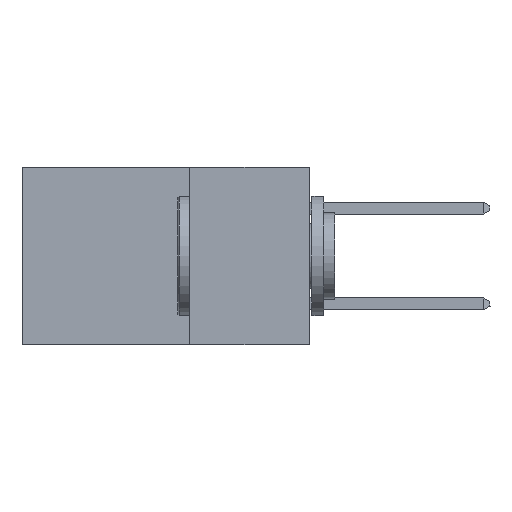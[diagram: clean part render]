
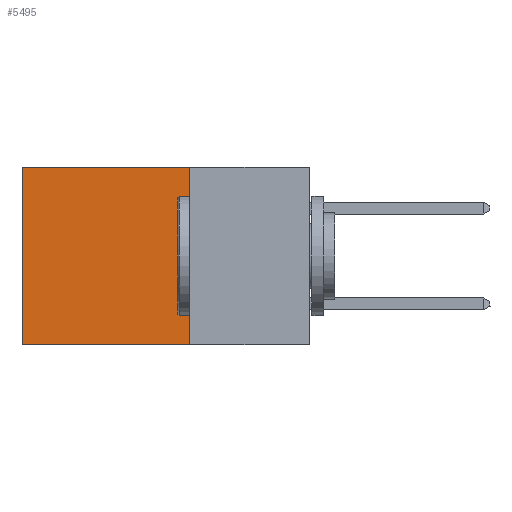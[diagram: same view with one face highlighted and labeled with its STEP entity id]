
A CAD part, left-side view. The second image highlights one B-rep face of the part: STEP entity #5495.
In plain terms, the highlighted planar face has unit normal (-1, 0, 0).
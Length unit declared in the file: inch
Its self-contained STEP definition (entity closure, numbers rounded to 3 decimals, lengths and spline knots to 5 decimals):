
#528 = EDGE_CURVE ( 'NONE', #16520, #16478, #780, .T. ) ;
#649 = EDGE_CURVE ( 'NONE', #1095, #3772, #18748, .T. ) ;
#780 = LINE ( 'NONE', #14561, #8374 ) ;
#1095 = VERTEX_POINT ( 'NONE', #7505 ) ;
#1180 = FACE_OUTER_BOUND ( 'NONE', #7968, .T. ) ;
#1362 = VECTOR ( 'NONE', #8903, 39.37008 ) ;
#2975 = DIRECTION ( 'NONE',  ( 0., 0., -1. ) ) ;
#3085 = AXIS2_PLACEMENT_3D ( 'NONE', #8882, #11912, #2975 ) ;
#3216 = ORIENTED_EDGE ( 'NONE', *, *, #11166, .F. ) ;
#3232 = LINE ( 'NONE', #18200, #10218 ) ;
#3411 = DIRECTION ( 'NONE',  ( 0., 0., -1. ) ) ;
#3772 = VERTEX_POINT ( 'NONE', #7283 ) ;
#5495 = ADVANCED_FACE ( 'NONE', ( #1180 ), #19245, .F. ) ;
#5923 = LINE ( 'NONE', #7429, #1362 ) ;
#7283 = CARTESIAN_POINT ( 'NONE',  ( 0.2875, 0.6, 0. ) ) ;
#7429 = CARTESIAN_POINT ( 'NONE',  ( 0.2875, 0.6, 0. ) ) ;
#7505 = CARTESIAN_POINT ( 'NONE',  ( 0.2875, 0.25, 0. ) ) ;
#7968 = EDGE_LOOP ( 'NONE', ( #13463, #12805, #3216, #14004 ) ) ;
#8374 = VECTOR ( 'NONE', #14510, 39.37008 ) ;
#8882 = CARTESIAN_POINT ( 'NONE',  ( 0.2875, 0.25, 0. ) ) ;
#8903 = DIRECTION ( 'NONE',  ( 0., 0., -1. ) ) ;
#10218 = VECTOR ( 'NONE', #3411, 39.37008 ) ;
#11166 = EDGE_CURVE ( 'NONE', #1095, #16520, #3232, .T. ) ;
#11912 = DIRECTION ( 'NONE',  ( 1., 0., 0. ) ) ;
#12805 = ORIENTED_EDGE ( 'NONE', *, *, #528, .F. ) ;
#12934 = DIRECTION ( 'NONE',  ( 0., 1., 0. ) ) ;
#13030 = CARTESIAN_POINT ( 'NONE',  ( 0.2875, 0.25, 0. ) ) ;
#13463 = ORIENTED_EDGE ( 'NONE', *, *, #18597, .T. ) ;
#13939 = VECTOR ( 'NONE', #12934, 39.37008 ) ;
#14004 = ORIENTED_EDGE ( 'NONE', *, *, #649, .T. ) ;
#14232 = CARTESIAN_POINT ( 'NONE',  ( 0.2875, 0.25, -0.37 ) ) ;
#14510 = DIRECTION ( 'NONE',  ( 0., 1., 0. ) ) ;
#14561 = CARTESIAN_POINT ( 'NONE',  ( 0.2875, 0.25, -0.37 ) ) ;
#15646 = CARTESIAN_POINT ( 'NONE',  ( 0.2875, 0.6, -0.37 ) ) ;
#16478 = VERTEX_POINT ( 'NONE', #15646 ) ;
#16520 = VERTEX_POINT ( 'NONE', #14232 ) ;
#18200 = CARTESIAN_POINT ( 'NONE',  ( 0.2875, 0.25, 0. ) ) ;
#18597 = EDGE_CURVE ( 'NONE', #3772, #16478, #5923, .T. ) ;
#18748 = LINE ( 'NONE', #13030, #13939 ) ;
#19245 = PLANE ( 'NONE',  #3085 ) ;
